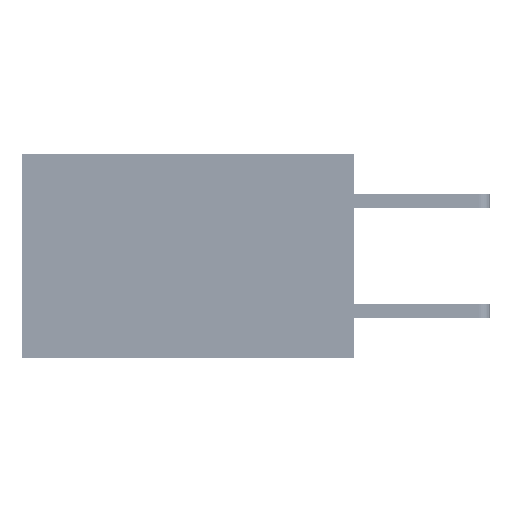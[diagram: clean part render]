
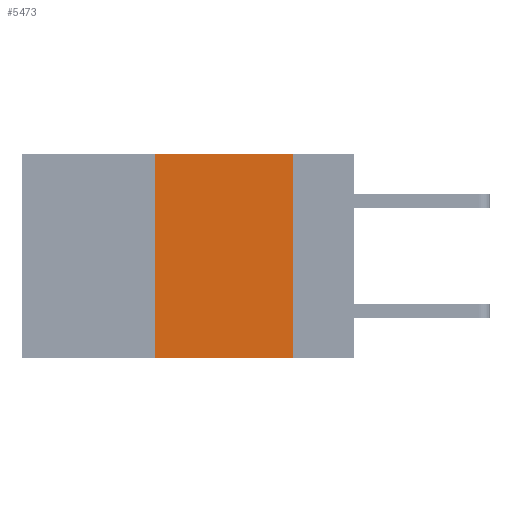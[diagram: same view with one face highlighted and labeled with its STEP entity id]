
A CAD part, left-side view. The second image highlights one B-rep face of the part: STEP entity #5473.
In plain terms, the highlighted planar face has unit normal (-1, 0, 0).
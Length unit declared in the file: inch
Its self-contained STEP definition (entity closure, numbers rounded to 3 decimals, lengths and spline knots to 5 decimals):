
#1200 = EDGE_CURVE ( 'NONE', #13181, #43335, #23179, .T. ) ;
#4727 = PLANE ( 'NONE',  #11829 ) ;
#5473 = ADVANCED_FACE ( 'NONE', ( #28279 ), #4727, .F. ) ;
#6147 = LINE ( 'NONE', #10284, #45329 ) ;
#8625 = EDGE_LOOP ( 'NONE', ( #25280, #19592, #17385, #50688 ) ) ;
#9994 = VERTEX_POINT ( 'NONE', #38413 ) ;
#10284 = CARTESIAN_POINT ( 'NONE',  ( 0., 0.11, 0. ) ) ;
#10745 = CARTESIAN_POINT ( 'NONE',  ( 0., 0.6, 0. ) ) ;
#11498 = CARTESIAN_POINT ( 'NONE',  ( 0., 0.36, 0. ) ) ;
#11829 = AXIS2_PLACEMENT_3D ( 'NONE', #16100, #20535, #27765 ) ;
#13181 = VERTEX_POINT ( 'NONE', #11498 ) ;
#13330 = VECTOR ( 'NONE', #27548, 39.37008 ) ;
#14172 = DIRECTION ( 'NONE',  ( 0., 0., -1. ) ) ;
#16100 = CARTESIAN_POINT ( 'NONE',  ( 0., 0.6, 0. ) ) ;
#17385 = ORIENTED_EDGE ( 'NONE', *, *, #42475, .F. ) ;
#19592 = ORIENTED_EDGE ( 'NONE', *, *, #1200, .F. ) ;
#20535 = DIRECTION ( 'NONE',  ( 1., 0., 0. ) ) ;
#23179 = LINE ( 'NONE', #10745, #39159 ) ;
#23187 = CARTESIAN_POINT ( 'NONE',  ( 0., 0.36, -0.37 ) ) ;
#23290 = CARTESIAN_POINT ( 'NONE',  ( 0., 0.6, -0.37 ) ) ;
#23673 = CARTESIAN_POINT ( 'NONE',  ( 0., 0.36, 0. ) ) ;
#25280 = ORIENTED_EDGE ( 'NONE', *, *, #34971, .F. ) ;
#27377 = VECTOR ( 'NONE', #30569, 39.37008 ) ;
#27548 = DIRECTION ( 'NONE',  ( 0., 0., 1. ) ) ;
#27765 = DIRECTION ( 'NONE',  ( 0., 0., -1. ) ) ;
#28279 = FACE_OUTER_BOUND ( 'NONE', #8625, .T. ) ;
#29299 = CARTESIAN_POINT ( 'NONE',  ( 0., 0.11, 0. ) ) ;
#29680 = LINE ( 'NONE', #23673, #13330 ) ;
#30569 = DIRECTION ( 'NONE',  ( 0., -1., 0. ) ) ;
#34471 = LINE ( 'NONE', #23290, #27377 ) ;
#34971 = EDGE_CURVE ( 'NONE', #43335, #9994, #6147, .T. ) ;
#38413 = CARTESIAN_POINT ( 'NONE',  ( 0., 0.11, -0.37 ) ) ;
#39159 = VECTOR ( 'NONE', #50138, 39.37008 ) ;
#42475 = EDGE_CURVE ( 'NONE', #44424, #13181, #29680, .T. ) ;
#43335 = VERTEX_POINT ( 'NONE', #29299 ) ;
#44424 = VERTEX_POINT ( 'NONE', #23187 ) ;
#45329 = VECTOR ( 'NONE', #14172, 39.37008 ) ;
#50138 = DIRECTION ( 'NONE',  ( 0., -1., 0. ) ) ;
#50521 = EDGE_CURVE ( 'NONE', #44424, #9994, #34471, .T. ) ;
#50688 = ORIENTED_EDGE ( 'NONE', *, *, #50521, .T. ) ;
